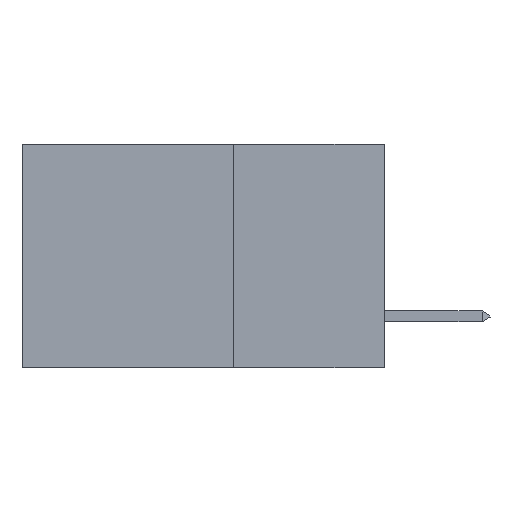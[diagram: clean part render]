
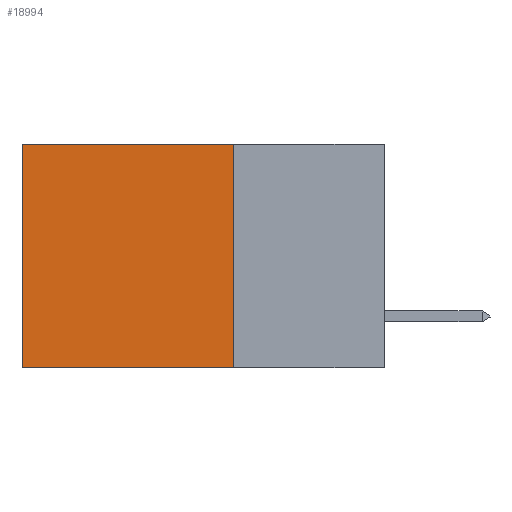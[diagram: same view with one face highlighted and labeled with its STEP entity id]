
A CAD part, left-side view. The second image highlights one B-rep face of the part: STEP entity #18994.
In plain terms, the highlighted planar face has unit normal (-1, 0, 0).
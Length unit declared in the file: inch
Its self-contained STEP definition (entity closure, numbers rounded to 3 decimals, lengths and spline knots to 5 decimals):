
#1069 = EDGE_CURVE ( 'NONE', #1362, #13494, #10614, .T. ) ;
#1362 = VERTEX_POINT ( 'NONE', #1480 ) ;
#1480 = CARTESIAN_POINT ( 'NONE',  ( 0.2875, 0.25, 0. ) ) ;
#2719 = DIRECTION ( 'NONE',  ( 0., 1., 0. ) ) ;
#2941 = VERTEX_POINT ( 'NONE', #11139 ) ;
#3169 = CARTESIAN_POINT ( 'NONE',  ( 0.2875, 0.6, -0.37 ) ) ;
#4130 = DIRECTION ( 'NONE',  ( 1., 0., 0. ) ) ;
#5618 = VECTOR ( 'NONE', #2719, 39.37008 ) ;
#5728 = DIRECTION ( 'NONE',  ( 0., 0., -1. ) ) ;
#5860 = PLANE ( 'NONE',  #14749 ) ;
#7269 = VECTOR ( 'NONE', #8750, 39.37008 ) ;
#7422 = CARTESIAN_POINT ( 'NONE',  ( 0.2875, 0.25, 0. ) ) ;
#7472 = CARTESIAN_POINT ( 'NONE',  ( 0.2875, 0.25, -0.37 ) ) ;
#7750 = VERTEX_POINT ( 'NONE', #3169 ) ;
#8554 = CARTESIAN_POINT ( 'NONE',  ( 0.2875, 0.25, -0.37 ) ) ;
#8750 = DIRECTION ( 'NONE',  ( 0., 0., -1. ) ) ;
#9373 = LINE ( 'NONE', #13093, #14146 ) ;
#10614 = LINE ( 'NONE', #11768, #7269 ) ;
#10658 = FACE_OUTER_BOUND ( 'NONE', #16928, .T. ) ;
#11139 = CARTESIAN_POINT ( 'NONE',  ( 0.2875, 0.6, 0. ) ) ;
#11240 = ORIENTED_EDGE ( 'NONE', *, *, #13963, .T. ) ;
#11352 = DIRECTION ( 'NONE',  ( 0., 0., -1. ) ) ;
#11766 = ORIENTED_EDGE ( 'NONE', *, *, #1069, .F. ) ;
#11768 = CARTESIAN_POINT ( 'NONE',  ( 0.2875, 0.25, 0. ) ) ;
#12074 = ORIENTED_EDGE ( 'NONE', *, *, #18539, .F. ) ;
#13084 = LINE ( 'NONE', #7472, #5618 ) ;
#13093 = CARTESIAN_POINT ( 'NONE',  ( 0.2875, 0.6, 0. ) ) ;
#13460 = DIRECTION ( 'NONE',  ( 0., 1., 0. ) ) ;
#13494 = VERTEX_POINT ( 'NONE', #8554 ) ;
#13963 = EDGE_CURVE ( 'NONE', #1362, #2941, #16576, .T. ) ;
#14146 = VECTOR ( 'NONE', #11352, 39.37008 ) ;
#14540 = ORIENTED_EDGE ( 'NONE', *, *, #14931, .T. ) ;
#14749 = AXIS2_PLACEMENT_3D ( 'NONE', #7422, #4130, #5728 ) ;
#14931 = EDGE_CURVE ( 'NONE', #2941, #7750, #9373, .T. ) ;
#16445 = CARTESIAN_POINT ( 'NONE',  ( 0.2875, 0.25, 0. ) ) ;
#16576 = LINE ( 'NONE', #16445, #17773 ) ;
#16928 = EDGE_LOOP ( 'NONE', ( #14540, #12074, #11766, #11240 ) ) ;
#17773 = VECTOR ( 'NONE', #13460, 39.37008 ) ;
#18539 = EDGE_CURVE ( 'NONE', #13494, #7750, #13084, .T. ) ;
#18994 = ADVANCED_FACE ( 'NONE', ( #10658 ), #5860, .F. ) ;
